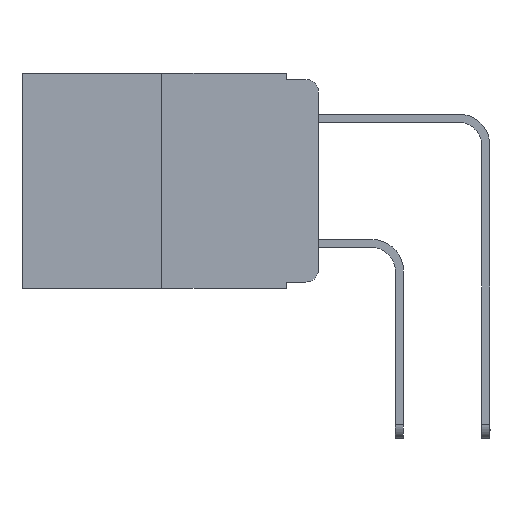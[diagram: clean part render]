
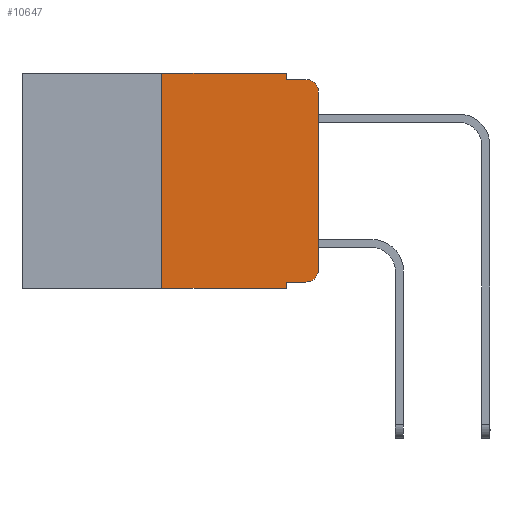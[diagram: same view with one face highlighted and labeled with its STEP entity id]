
A CAD part, left-side view. The second image highlights one B-rep face of the part: STEP entity #10647.
In plain terms, the highlighted planar face has unit normal (-1, 0, 0).
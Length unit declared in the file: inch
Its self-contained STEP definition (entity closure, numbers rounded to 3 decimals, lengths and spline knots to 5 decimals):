
#840 = FACE_OUTER_BOUND ( 'NONE', #5678, .T. ) ;
#927 = VERTEX_POINT ( 'NONE', #7985 ) ;
#970 = LINE ( 'NONE', #21047, #13373 ) ;
#1377 = CARTESIAN_POINT ( 'NONE',  ( 0., 0.051, 0. ) ) ;
#1735 = DIRECTION ( 'NONE',  ( 0., 0., -1. ) ) ;
#2970 = EDGE_CURVE ( 'NONE', #17706, #26643, #25454, .T. ) ;
#3407 = EDGE_CURVE ( 'NONE', #10576, #15763, #15329, .T. ) ;
#4026 = ORIENTED_EDGE ( 'NONE', *, *, #12670, .F. ) ;
#4100 = EDGE_CURVE ( 'NONE', #927, #6852, #24379, .T. ) ;
#4426 = CARTESIAN_POINT ( 'NONE',  ( 0., 0.051, -0.333 ) ) ;
#4866 = DIRECTION ( 'NONE',  ( 0., 0., 1. ) ) ;
#5411 = PLANE ( 'NONE',  #8551 ) ;
#5580 = DIRECTION ( 'NONE',  ( 0., -1., 0. ) ) ;
#5678 = EDGE_LOOP ( 'NONE', ( #13539, #18072, #12172, #14584, #21448, #12223, #16804, #4026, #13680, #6462 ) ) ;
#6462 = ORIENTED_EDGE ( 'NONE', *, *, #25559, .T. ) ;
#6852 = VERTEX_POINT ( 'NONE', #13018 ) ;
#6855 = DIRECTION ( 'NONE',  ( 0., -1., 0. ) ) ;
#7087 = DIRECTION ( 'NONE',  ( 0., 0., 1. ) ) ;
#7166 = CARTESIAN_POINT ( 'NONE',  ( 0., 0., 0. ) ) ;
#7401 = CARTESIAN_POINT ( 'NONE',  ( 0., 0.051, -0.01 ) ) ;
#7492 = CARTESIAN_POINT ( 'NONE',  ( 0., 0.02, -0.313 ) ) ;
#7584 = VECTOR ( 'NONE', #5580, 39.37008 ) ;
#7727 = EDGE_CURVE ( 'NONE', #18498, #23976, #970, .T. ) ;
#7985 = CARTESIAN_POINT ( 'NONE',  ( 0., 0., -0.03 ) ) ;
#8109 = CARTESIAN_POINT ( 'NONE',  ( 0., 0.25, 0. ) ) ;
#8138 = VECTOR ( 'NONE', #4866, 39.37008 ) ;
#8231 = CIRCLE ( 'NONE', #18757, 0.02 ) ;
#8551 = AXIS2_PLACEMENT_3D ( 'NONE', #22062, #26318, #13685 ) ;
#9317 = VECTOR ( 'NONE', #12031, 39.37008 ) ;
#10576 = VERTEX_POINT ( 'NONE', #17407 ) ;
#10647 = ADVANCED_FACE ( 'NONE', ( #840 ), #5411, .F. ) ;
#11258 = CARTESIAN_POINT ( 'NONE',  ( 0., 0.051, 0. ) ) ;
#11749 = CARTESIAN_POINT ( 'NONE',  ( 0., 0.473, -0.343 ) ) ;
#11754 = DIRECTION ( 'NONE',  ( 0., 0., -1. ) ) ;
#11778 = VECTOR ( 'NONE', #21005, 39.37008 ) ;
#12031 = DIRECTION ( 'NONE',  ( 0., 0., -1. ) ) ;
#12172 = ORIENTED_EDGE ( 'NONE', *, *, #25596, .F. ) ;
#12223 = ORIENTED_EDGE ( 'NONE', *, *, #13703, .F. ) ;
#12468 = DIRECTION ( 'NONE',  ( -1., 0., 0. ) ) ;
#12670 = EDGE_CURVE ( 'NONE', #18498, #15763, #16146, .T. ) ;
#13018 = CARTESIAN_POINT ( 'NONE',  ( 0., 0.02, -0.01 ) ) ;
#13104 = LINE ( 'NONE', #7401, #7584 ) ;
#13373 = VECTOR ( 'NONE', #6855, 39.37008 ) ;
#13468 = VERTEX_POINT ( 'NONE', #22817 ) ;
#13539 = ORIENTED_EDGE ( 'NONE', *, *, #16808, .T. ) ;
#13678 = LINE ( 'NONE', #7166, #8138 ) ;
#13680 = ORIENTED_EDGE ( 'NONE', *, *, #7727, .T. ) ;
#13684 = VECTOR ( 'NONE', #22227, 39.37008 ) ;
#13685 = DIRECTION ( 'NONE',  ( 0., 0., -1. ) ) ;
#13703 = EDGE_CURVE ( 'NONE', #10576, #17706, #23636, .T. ) ;
#14282 = CARTESIAN_POINT ( 'NONE',  ( 0., 0.051, 0. ) ) ;
#14584 = ORIENTED_EDGE ( 'NONE', *, *, #15487, .F. ) ;
#14841 = VECTOR ( 'NONE', #7087, 39.37008 ) ;
#15329 = LINE ( 'NONE', #11749, #13684 ) ;
#15345 = CARTESIAN_POINT ( 'NONE',  ( 0., 0.051, -0.343 ) ) ;
#15441 = CARTESIAN_POINT ( 'NONE',  ( 0., 0.25, 0. ) ) ;
#15487 = EDGE_CURVE ( 'NONE', #26643, #13468, #24809, .T. ) ;
#15763 = VERTEX_POINT ( 'NONE', #15345 ) ;
#16146 = LINE ( 'NONE', #1377, #9317 ) ;
#16804 = ORIENTED_EDGE ( 'NONE', *, *, #3407, .T. ) ;
#16808 = EDGE_CURVE ( 'NONE', #17209, #927, #13678, .T. ) ;
#16959 = CARTESIAN_POINT ( 'NONE',  ( 0., 0., -0.313 ) ) ;
#17209 = VERTEX_POINT ( 'NONE', #16959 ) ;
#17407 = CARTESIAN_POINT ( 'NONE',  ( 0., 0.25, -0.343 ) ) ;
#17706 = VERTEX_POINT ( 'NONE', #8109 ) ;
#17839 = CARTESIAN_POINT ( 'NONE',  ( 0., 0.02, -0.333 ) ) ;
#18072 = ORIENTED_EDGE ( 'NONE', *, *, #4100, .T. ) ;
#18498 = VERTEX_POINT ( 'NONE', #4426 ) ;
#18534 = CARTESIAN_POINT ( 'NONE',  ( 0., 0.473, 0. ) ) ;
#18757 = AXIS2_PLACEMENT_3D ( 'NONE', #7492, #20073, #11754 ) ;
#20073 = DIRECTION ( 'NONE',  ( -1., 0., 0. ) ) ;
#20691 = CARTESIAN_POINT ( 'NONE',  ( 0., 0.02, -0.03 ) ) ;
#20901 = VECTOR ( 'NONE', #22898, 39.37008 ) ;
#21005 = DIRECTION ( 'NONE',  ( 0., 0., -1. ) ) ;
#21047 = CARTESIAN_POINT ( 'NONE',  ( 0., 0.051, -0.333 ) ) ;
#21448 = ORIENTED_EDGE ( 'NONE', *, *, #2970, .F. ) ;
#22062 = CARTESIAN_POINT ( 'NONE',  ( 0., 0.473, 0. ) ) ;
#22206 = AXIS2_PLACEMENT_3D ( 'NONE', #20691, #12468, #1735 ) ;
#22227 = DIRECTION ( 'NONE',  ( 0., -1., 0. ) ) ;
#22817 = CARTESIAN_POINT ( 'NONE',  ( 0., 0.051, -0.01 ) ) ;
#22898 = DIRECTION ( 'NONE',  ( 0., -1., 0. ) ) ;
#23636 = LINE ( 'NONE', #15441, #14841 ) ;
#23976 = VERTEX_POINT ( 'NONE', #17839 ) ;
#24379 = CIRCLE ( 'NONE', #22206, 0.02 ) ;
#24809 = LINE ( 'NONE', #14282, #11778 ) ;
#25454 = LINE ( 'NONE', #18534, #20901 ) ;
#25559 = EDGE_CURVE ( 'NONE', #23976, #17209, #8231, .T. ) ;
#25596 = EDGE_CURVE ( 'NONE', #13468, #6852, #13104, .T. ) ;
#26318 = DIRECTION ( 'NONE',  ( 1., 0., 0. ) ) ;
#26643 = VERTEX_POINT ( 'NONE', #11258 ) ;
